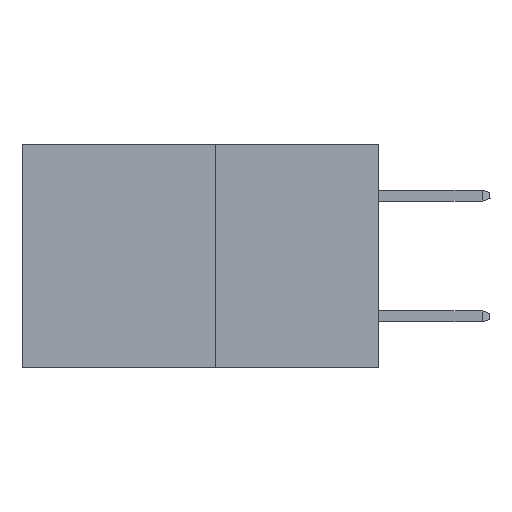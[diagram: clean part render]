
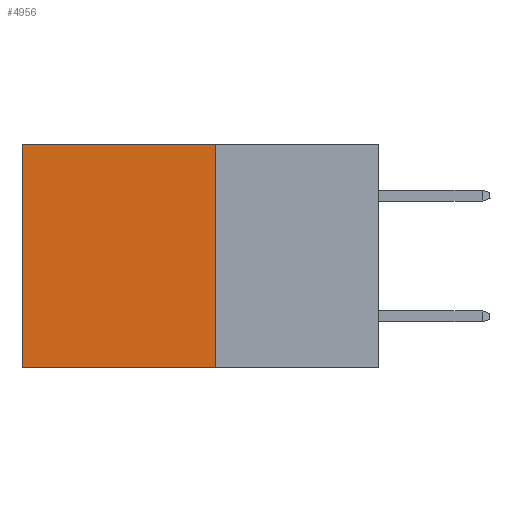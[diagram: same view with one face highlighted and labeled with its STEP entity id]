
A CAD part, left-side view. The second image highlights one B-rep face of the part: STEP entity #4956.
In plain terms, the highlighted planar face has unit normal (-1, 0, 0).
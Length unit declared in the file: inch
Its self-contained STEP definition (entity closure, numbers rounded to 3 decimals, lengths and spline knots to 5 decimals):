
#69 = VERTEX_POINT ( 'NONE', #1735 ) ;
#270 = CARTESIAN_POINT ( 'NONE',  ( 0.277, 0.59, -0.37 ) ) ;
#774 = DIRECTION ( 'NONE',  ( 0., 0., -1. ) ) ;
#884 = DIRECTION ( 'NONE',  ( 0., 1., 0. ) ) ;
#971 = VERTEX_POINT ( 'NONE', #270 ) ;
#1298 = DIRECTION ( 'NONE',  ( 1., 0., 0. ) ) ;
#1519 = FACE_OUTER_BOUND ( 'NONE', #9171, .T. ) ;
#1555 = VECTOR ( 'NONE', #4641, 39.37008 ) ;
#1735 = CARTESIAN_POINT ( 'NONE',  ( 0.277, 0.27, -0.37 ) ) ;
#2076 = ORIENTED_EDGE ( 'NONE', *, *, #2716, .T. ) ;
#2227 = VECTOR ( 'NONE', #4773, 39.37008 ) ;
#2468 = CARTESIAN_POINT ( 'NONE',  ( 0.277, 0.27, 0. ) ) ;
#2716 = EDGE_CURVE ( 'NONE', #10279, #5867, #7614, .T. ) ;
#2783 = LINE ( 'NONE', #14545, #8609 ) ;
#2857 = ORIENTED_EDGE ( 'NONE', *, *, #11250, .F. ) ;
#4073 = ORIENTED_EDGE ( 'NONE', *, *, #11944, .F. ) ;
#4641 = DIRECTION ( 'NONE',  ( 0., 1., 0. ) ) ;
#4773 = DIRECTION ( 'NONE',  ( 0., 0., -1. ) ) ;
#4836 = AXIS2_PLACEMENT_3D ( 'NONE', #6038, #1298, #774 ) ;
#4956 = ADVANCED_FACE ( 'NONE', ( #1519 ), #5919, .F. ) ;
#5867 = VERTEX_POINT ( 'NONE', #13043 ) ;
#5919 = PLANE ( 'NONE',  #4836 ) ;
#6038 = CARTESIAN_POINT ( 'NONE',  ( 0.277, 0.27, -0.37 ) ) ;
#6590 = VECTOR ( 'NONE', #10479, 39.37008 ) ;
#6883 = ORIENTED_EDGE ( 'NONE', *, *, #13357, .T. ) ;
#6949 = LINE ( 'NONE', #9323, #6590 ) ;
#7614 = LINE ( 'NONE', #11495, #1555 ) ;
#8609 = VECTOR ( 'NONE', #884, 39.37008 ) ;
#9171 = EDGE_LOOP ( 'NONE', ( #6883, #4073, #2857, #2076 ) ) ;
#9323 = CARTESIAN_POINT ( 'NONE',  ( 0.277, 0.27, -0.37 ) ) ;
#10279 = VERTEX_POINT ( 'NONE', #2468 ) ;
#10479 = DIRECTION ( 'NONE',  ( 0., 0., -1. ) ) ;
#11250 = EDGE_CURVE ( 'NONE', #10279, #69, #6949, .T. ) ;
#11495 = CARTESIAN_POINT ( 'NONE',  ( 0.277, 0.27, 0. ) ) ;
#11944 = EDGE_CURVE ( 'NONE', #69, #971, #2783, .T. ) ;
#13043 = CARTESIAN_POINT ( 'NONE',  ( 0.277, 0.59, 0. ) ) ;
#13357 = EDGE_CURVE ( 'NONE', #5867, #971, #14373, .T. ) ;
#13923 = CARTESIAN_POINT ( 'NONE',  ( 0.277, 0.59, -0.37 ) ) ;
#14373 = LINE ( 'NONE', #13923, #2227 ) ;
#14545 = CARTESIAN_POINT ( 'NONE',  ( 0.277, 0.27, -0.37 ) ) ;
